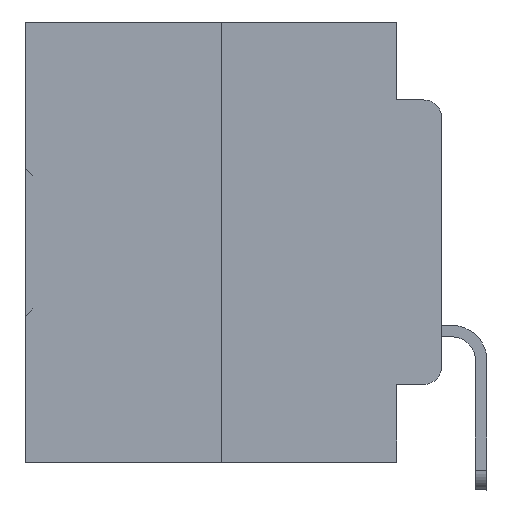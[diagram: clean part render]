
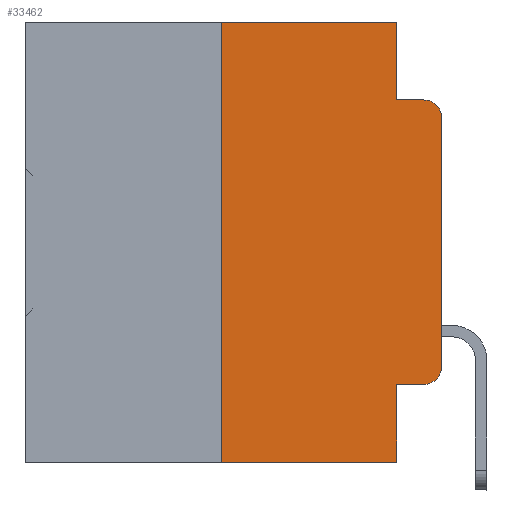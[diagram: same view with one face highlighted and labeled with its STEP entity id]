
A CAD part, left-side view. The second image highlights one B-rep face of the part: STEP entity #33462.
In plain terms, the highlighted planar face has unit normal (-1, 0, 0).
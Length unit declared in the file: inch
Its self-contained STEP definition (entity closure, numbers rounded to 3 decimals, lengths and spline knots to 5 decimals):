
#1026 = DIRECTION ( 'NONE',  ( 0., 0., 1. ) ) ;
#1647 = EDGE_LOOP ( 'NONE', ( #15077, #18293, #10928, #9715, #20330, #6369, #16176, #9781, #1727, #26102 ) ) ;
#1727 = ORIENTED_EDGE ( 'NONE', *, *, #34543, .T. ) ;
#2032 = EDGE_CURVE ( 'NONE', #28413, #4509, #21538, .T. ) ;
#2354 = VERTEX_POINT ( 'NONE', #5241 ) ;
#2455 = EDGE_CURVE ( 'NONE', #14828, #14195, #4495, .T. ) ;
#3155 = DIRECTION ( 'NONE',  ( 0., 0., -1. ) ) ;
#3222 = CARTESIAN_POINT ( 'NONE',  ( 0., 0.02, -0.4115 ) ) ;
#3816 = VERTEX_POINT ( 'NONE', #13464 ) ;
#4258 = AXIS2_PLACEMENT_3D ( 'NONE', #15510, #9794, #15403 ) ;
#4301 = DIRECTION ( 'NONE',  ( 0., -1., 0. ) ) ;
#4495 = CIRCLE ( 'NONE', #32082, 0.02 ) ;
#4509 = VERTEX_POINT ( 'NONE', #21326 ) ;
#5241 = CARTESIAN_POINT ( 'NONE',  ( 0., 0.051, 0. ) ) ;
#5441 = DIRECTION ( 'NONE',  ( 0., -1., 0. ) ) ;
#5850 = EDGE_CURVE ( 'NONE', #28413, #10619, #19953, .T. ) ;
#6065 = CARTESIAN_POINT ( 'NONE',  ( 0., 0., -0.3915 ) ) ;
#6191 = DIRECTION ( 'NONE',  ( 0., -1., 0. ) ) ;
#6369 = ORIENTED_EDGE ( 'NONE', *, *, #2032, .F. ) ;
#7144 = VECTOR ( 'NONE', #4301, 39.37008 ) ;
#7714 = LINE ( 'NONE', #28598, #32108 ) ;
#8194 = CARTESIAN_POINT ( 'NONE',  ( 0., 0.051, 0. ) ) ;
#8294 = VECTOR ( 'NONE', #24200, 39.37008 ) ;
#8985 = CARTESIAN_POINT ( 'NONE',  ( 0., 0.02, -0.3915 ) ) ;
#9715 = ORIENTED_EDGE ( 'NONE', *, *, #26585, .F. ) ;
#9781 = ORIENTED_EDGE ( 'NONE', *, *, #18929, .F. ) ;
#9794 = DIRECTION ( 'NONE',  ( 1., 0., 0. ) ) ;
#10010 = LINE ( 'NONE', #8194, #32724 ) ;
#10619 = VERTEX_POINT ( 'NONE', #22119 ) ;
#10654 = LINE ( 'NONE', #12367, #7144 ) ;
#10928 = ORIENTED_EDGE ( 'NONE', *, *, #16703, .F. ) ;
#11145 = VECTOR ( 'NONE', #1026, 39.37008 ) ;
#11349 = DIRECTION ( 'NONE',  ( 0., 0., -1. ) ) ;
#11508 = CARTESIAN_POINT ( 'NONE',  ( 0., 0.02, -0.1085 ) ) ;
#11909 = DIRECTION ( 'NONE',  ( -1., 0., 0. ) ) ;
#12364 = CIRCLE ( 'NONE', #14234, 0.02 ) ;
#12367 = CARTESIAN_POINT ( 'NONE',  ( 0., 0.051, -0.0885 ) ) ;
#13464 = CARTESIAN_POINT ( 'NONE',  ( 0., 0., -0.1085 ) ) ;
#13515 = LINE ( 'NONE', #21245, #8294 ) ;
#14195 = VERTEX_POINT ( 'NONE', #6065 ) ;
#14234 = AXIS2_PLACEMENT_3D ( 'NONE', #11508, #33906, #20135 ) ;
#14555 = CARTESIAN_POINT ( 'NONE',  ( 0., 0.473, -0.5 ) ) ;
#14828 = VERTEX_POINT ( 'NONE', #3222 ) ;
#15038 = DIRECTION ( 'NONE',  ( 0., -1., 0. ) ) ;
#15077 = ORIENTED_EDGE ( 'NONE', *, *, #28045, .T. ) ;
#15403 = DIRECTION ( 'NONE',  ( 0., 0., -1. ) ) ;
#15510 = CARTESIAN_POINT ( 'NONE',  ( 0., 0.473, 0. ) ) ;
#16176 = ORIENTED_EDGE ( 'NONE', *, *, #5850, .T. ) ;
#16703 = EDGE_CURVE ( 'NONE', #21171, #28559, #10654, .T. ) ;
#16968 = VECTOR ( 'NONE', #15038, 39.37008 ) ;
#18293 = ORIENTED_EDGE ( 'NONE', *, *, #20327, .T. ) ;
#18929 = EDGE_CURVE ( 'NONE', #19226, #10619, #10010, .T. ) ;
#19226 = VERTEX_POINT ( 'NONE', #35306 ) ;
#19953 = LINE ( 'NONE', #14555, #34769 ) ;
#20135 = DIRECTION ( 'NONE',  ( 0., 0., -1. ) ) ;
#20327 = EDGE_CURVE ( 'NONE', #3816, #28559, #12364, .T. ) ;
#20330 = ORIENTED_EDGE ( 'NONE', *, *, #27024, .F. ) ;
#20626 = CARTESIAN_POINT ( 'NONE',  ( 0., 0., 0. ) ) ;
#20979 = PLANE ( 'NONE',  #4258 ) ;
#21171 = VERTEX_POINT ( 'NONE', #32022 ) ;
#21245 = CARTESIAN_POINT ( 'NONE',  ( 0., 0.051, 0. ) ) ;
#21326 = CARTESIAN_POINT ( 'NONE',  ( 0., 0.25, 0. ) ) ;
#21538 = LINE ( 'NONE', #32416, #21971 ) ;
#21971 = VECTOR ( 'NONE', #26565, 39.37008 ) ;
#22119 = CARTESIAN_POINT ( 'NONE',  ( 0., 0.051, -0.5 ) ) ;
#24200 = DIRECTION ( 'NONE',  ( 0., 0., -1. ) ) ;
#26102 = ORIENTED_EDGE ( 'NONE', *, *, #2455, .T. ) ;
#26565 = DIRECTION ( 'NONE',  ( 0., 0., 1. ) ) ;
#26585 = EDGE_CURVE ( 'NONE', #2354, #21171, #13515, .T. ) ;
#27024 = EDGE_CURVE ( 'NONE', #4509, #2354, #32175, .T. ) ;
#27719 = LINE ( 'NONE', #20626, #11145 ) ;
#28045 = EDGE_CURVE ( 'NONE', #14195, #3816, #27719, .T. ) ;
#28413 = VERTEX_POINT ( 'NONE', #35357 ) ;
#28415 = CARTESIAN_POINT ( 'NONE',  ( 0., 0.02, -0.0885 ) ) ;
#28559 = VERTEX_POINT ( 'NONE', #28415 ) ;
#28574 = CARTESIAN_POINT ( 'NONE',  ( 0., 0.473, 0. ) ) ;
#28598 = CARTESIAN_POINT ( 'NONE',  ( 0., 0.051, -0.4115 ) ) ;
#32022 = CARTESIAN_POINT ( 'NONE',  ( 0., 0.051, -0.0885 ) ) ;
#32082 = AXIS2_PLACEMENT_3D ( 'NONE', #8985, #11909, #3155 ) ;
#32108 = VECTOR ( 'NONE', #6191, 39.37008 ) ;
#32175 = LINE ( 'NONE', #28574, #16968 ) ;
#32416 = CARTESIAN_POINT ( 'NONE',  ( 0., 0.25, 0. ) ) ;
#32724 = VECTOR ( 'NONE', #11349, 39.37008 ) ;
#33462 = ADVANCED_FACE ( 'NONE', ( #34750 ), #20979, .F. ) ;
#33906 = DIRECTION ( 'NONE',  ( -1., 0., 0. ) ) ;
#34543 = EDGE_CURVE ( 'NONE', #19226, #14828, #7714, .T. ) ;
#34750 = FACE_OUTER_BOUND ( 'NONE', #1647, .T. ) ;
#34769 = VECTOR ( 'NONE', #5441, 39.37008 ) ;
#35306 = CARTESIAN_POINT ( 'NONE',  ( 0., 0.051, -0.4115 ) ) ;
#35357 = CARTESIAN_POINT ( 'NONE',  ( 0., 0.25, -0.5 ) ) ;
